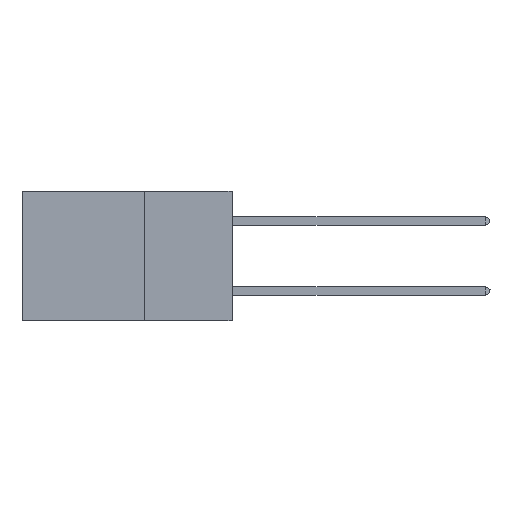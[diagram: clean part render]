
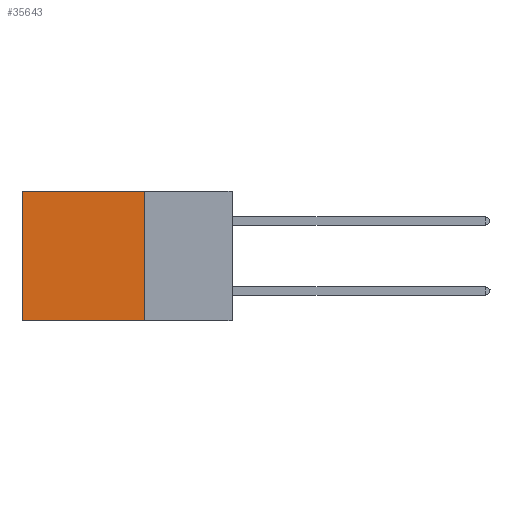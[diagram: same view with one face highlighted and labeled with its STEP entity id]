
A CAD part, left-side view. The second image highlights one B-rep face of the part: STEP entity #35643.
In plain terms, the highlighted planar face has unit normal (-1, 0, 0).
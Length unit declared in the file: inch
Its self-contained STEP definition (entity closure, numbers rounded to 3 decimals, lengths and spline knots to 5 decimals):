
#3279 = PLANE ( 'NONE',  #34198 ) ;
#3465 = ORIENTED_EDGE ( 'NONE', *, *, #3642, .T. ) ;
#3473 = DIRECTION ( 'NONE',  ( 1., 0., 0. ) ) ;
#3642 = EDGE_CURVE ( 'NONE', #30321, #6726, #35376, .T. ) ;
#4342 = CARTESIAN_POINT ( 'NONE',  ( 0.2875, 0.25, 0. ) ) ;
#4394 = CARTESIAN_POINT ( 'NONE',  ( 0.2875, 0.25, -0.37 ) ) ;
#5018 = CARTESIAN_POINT ( 'NONE',  ( 0.2875, 0.6, -0.37 ) ) ;
#5117 = VERTEX_POINT ( 'NONE', #9917 ) ;
#6726 = VERTEX_POINT ( 'NONE', #5018 ) ;
#7177 = LINE ( 'NONE', #4342, #27040 ) ;
#9502 = CARTESIAN_POINT ( 'NONE',  ( 0.2875, 0.6, 0. ) ) ;
#9917 = CARTESIAN_POINT ( 'NONE',  ( 0.2875, 0.25, 0. ) ) ;
#11627 = DIRECTION ( 'NONE',  ( 0., 1., 0. ) ) ;
#13676 = ORIENTED_EDGE ( 'NONE', *, *, #25107, .F. ) ;
#15135 = CARTESIAN_POINT ( 'NONE',  ( 0.2875, 0.6, 0. ) ) ;
#15475 = EDGE_LOOP ( 'NONE', ( #3465, #13676, #24957, #27786 ) ) ;
#15856 = DIRECTION ( 'NONE',  ( 0., 0., -1. ) ) ;
#16466 = EDGE_CURVE ( 'NONE', #5117, #22970, #7177, .T. ) ;
#18376 = CARTESIAN_POINT ( 'NONE',  ( 0.2875, 0.25, 0. ) ) ;
#19899 = VECTOR ( 'NONE', #11627, 39.37008 ) ;
#21019 = DIRECTION ( 'NONE',  ( 0., 0., -1. ) ) ;
#22970 = VERTEX_POINT ( 'NONE', #4394 ) ;
#24153 = VECTOR ( 'NONE', #21019, 39.37008 ) ;
#24957 = ORIENTED_EDGE ( 'NONE', *, *, #16466, .F. ) ;
#25107 = EDGE_CURVE ( 'NONE', #22970, #6726, #26426, .T. ) ;
#26317 = FACE_OUTER_BOUND ( 'NONE', #15475, .T. ) ;
#26426 = LINE ( 'NONE', #34743, #34991 ) ;
#26639 = EDGE_CURVE ( 'NONE', #5117, #30321, #28609, .T. ) ;
#27040 = VECTOR ( 'NONE', #15856, 39.37008 ) ;
#27786 = ORIENTED_EDGE ( 'NONE', *, *, #26639, .T. ) ;
#28609 = LINE ( 'NONE', #31444, #19899 ) ;
#30321 = VERTEX_POINT ( 'NONE', #15135 ) ;
#31444 = CARTESIAN_POINT ( 'NONE',  ( 0.2875, 0.25, 0. ) ) ;
#32544 = DIRECTION ( 'NONE',  ( 0., 0., -1. ) ) ;
#34198 = AXIS2_PLACEMENT_3D ( 'NONE', #18376, #3473, #32544 ) ;
#34358 = DIRECTION ( 'NONE',  ( 0., 1., 0. ) ) ;
#34743 = CARTESIAN_POINT ( 'NONE',  ( 0.2875, 0.25, -0.37 ) ) ;
#34991 = VECTOR ( 'NONE', #34358, 39.37008 ) ;
#35376 = LINE ( 'NONE', #9502, #24153 ) ;
#35643 = ADVANCED_FACE ( 'NONE', ( #26317 ), #3279, .F. ) ;
